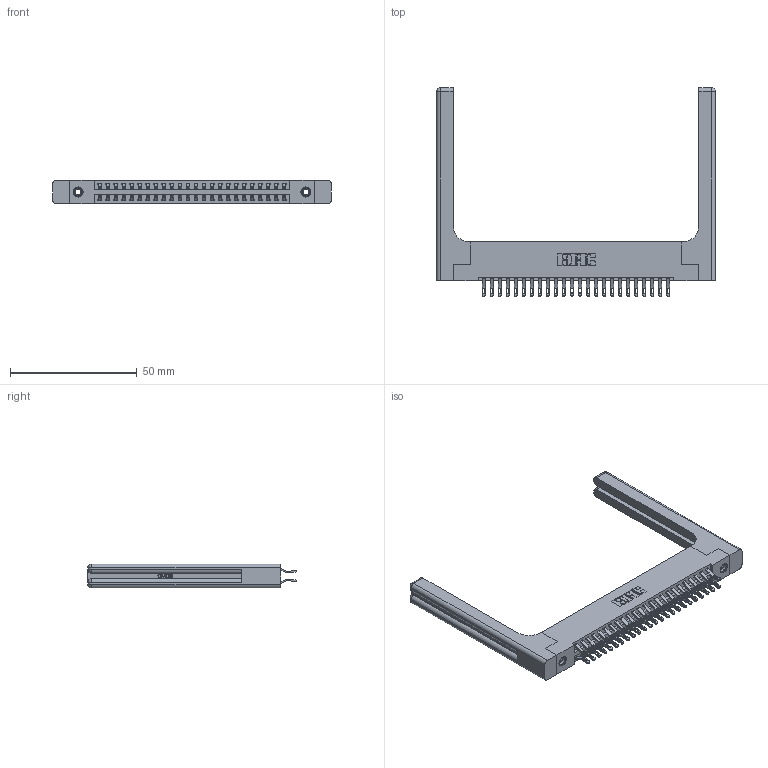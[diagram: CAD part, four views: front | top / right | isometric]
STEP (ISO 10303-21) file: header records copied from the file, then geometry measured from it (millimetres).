
FILE_DESCRIPTION (( 'STEP AP203' ), '1' );
FILE_NAME ('346-048-555-258.STEP', '2022-05-20T21:50:26', ( '' ), ( '' ), 'SwSTEP 2.0', 'SolidWorks 2020', '' );
FILE_SCHEMA (( 'CONFIG_CONTROL_DESIGN' ));
Length unit declared in the file: inch
Products named in the file (5): 346-220-058_345-220-058; 346-048-555-258; 345-292-001_555 Tail; 345-250-001_345-250-001-102; 346 Part_Flush Mounting Lugs - 0.156 Dia-TH
Assembly tree (53 placements, depth 2):
  346-048-555-258
    346 Part_Flush Mounting Lugs - 0.156 Dia-TH
    345-292-001_555 Tail  x48
    345-250-001_345-250-001-102  x2
    346-220-058_345-220-058  x2
Bounding box: 110.26 x 82.42 x 9.4 mm (x, y, z)
Volume: 18227.4 mm3; surface area: 19974.2 mm2
Topology: 53 solids, 53 shells, 3176 faces, 9815 edges, 6522 vertices
Faces by surface type: plane 1822, cylinder 1294, bspline 36, cone 12, sphere 8, torus 4
Entity records: 24010 total; most frequent: CARTESIAN_POINT 5029, ORIENTED_EDGE 3728, DIRECTION 3384, EDGE_CURVE 1864, LINE 1524, VECTOR 1524, VERTEX_POINT 1234, AXIS2_PLACEMENT_3D 930
